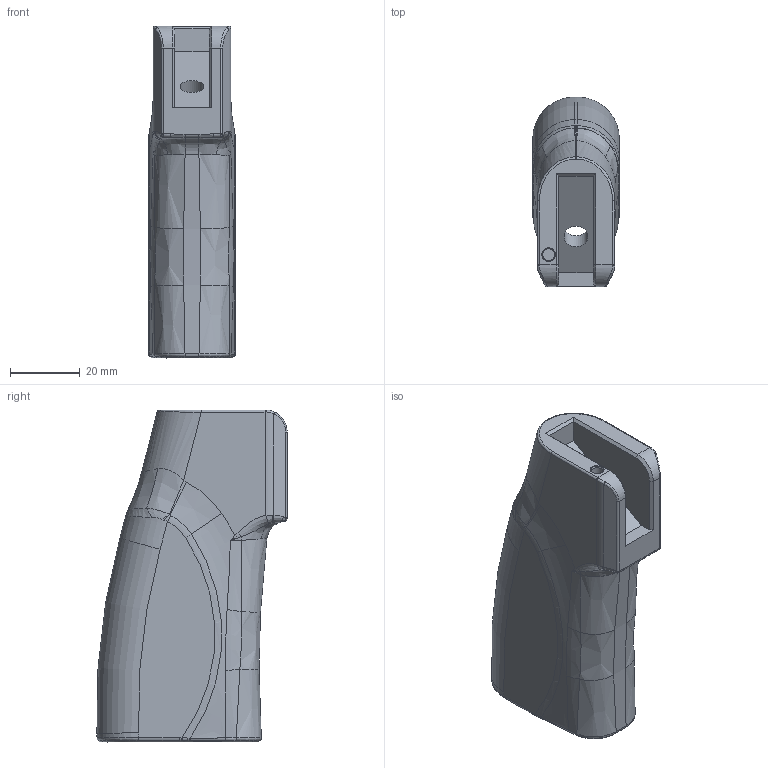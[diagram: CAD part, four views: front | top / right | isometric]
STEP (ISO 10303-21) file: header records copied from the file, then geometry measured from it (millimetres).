
FILE_DESCRIPTION(/* description */ (''),/* implementation_level */ '2;1');
FILE_NAME(/* name */ 'VertiGrip Lite.step',/* time_stamp */ '2021-10-15T02:07:45-04:00',/* author */ (''),/* organization */ (''),/* preprocessor_version */ 'ST-DEVELOPER v18.1',/* originating_system */ 'Autodesk Translation Framework v10.10.0.1391',/* authorisation */ '');
FILE_SCHEMA (('AUTOMOTIVE_DESIGN { 1 0 10303 214 3 1 1 }'));
Length unit declared in the file: millimetre
Products named in the file (1): VertiGrip Lite
Bounding box: 24.83 x 54.66 x 95.41 mm (x, y, z)
Volume: 44751.5 mm3; surface area: 21188.5 mm2
Topology: 1 solids, 1 shells, 373 faces, 911 edges, 539 vertices
Faces by surface type: bspline 221, torus 57, plane 46, cylinder 45, cone 4
Full cylindrical faces by diameter (mm): 3.4 x1, 6.8 x1, 15.489 x1
Entity records: 17153 total; most frequent: CARTESIAN_POINT 9667, ORIENTED_EDGE 1806, DIRECTION 1130, EDGE_CURVE 903, VERTEX_POINT 539, AXIS2_PLACEMENT_3D 475, B_SPLINE_CURVE_WITH_KNOTS 401, EDGE_LOOP 382
